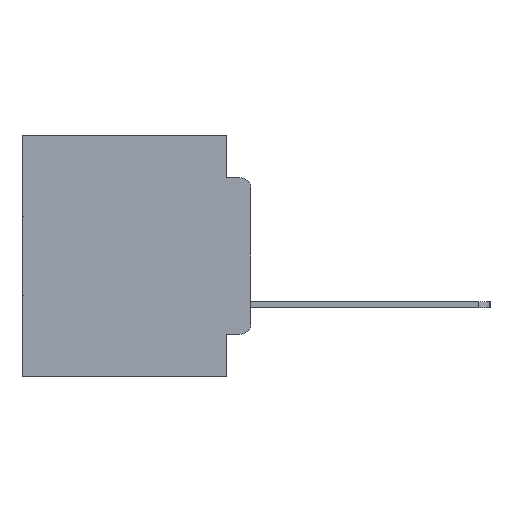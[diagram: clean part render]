
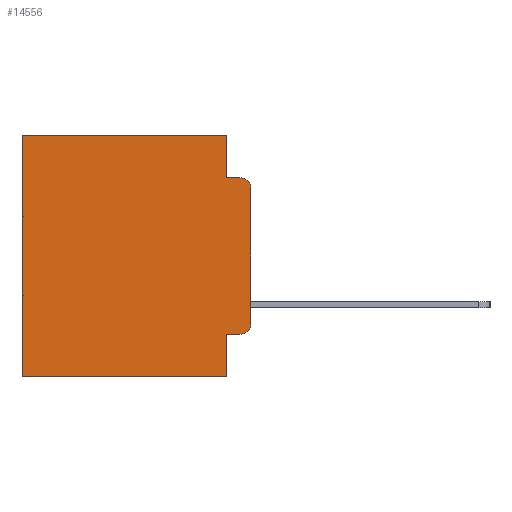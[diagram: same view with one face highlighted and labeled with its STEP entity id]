
A CAD part, left-side view. The second image highlights one B-rep face of the part: STEP entity #14556.
In plain terms, the highlighted planar face has unit normal (-1, 0, 0).
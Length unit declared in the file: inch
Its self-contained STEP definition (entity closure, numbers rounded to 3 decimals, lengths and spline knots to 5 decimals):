
#582 = DIRECTION ( 'NONE',  ( 0., 1., 0. ) ) ;
#583 = EDGE_CURVE ( 'NONE', #15715, #18864, #4426, .T. ) ;
#731 = DIRECTION ( 'NONE',  ( 0., 1., 0. ) ) ;
#733 = CARTESIAN_POINT ( 'NONE',  ( 0.298, 0.051, 0. ) ) ;
#895 = CARTESIAN_POINT ( 'NONE',  ( 0.298, 0., -0.1085 ) ) ;
#943 = VERTEX_POINT ( 'NONE', #2730 ) ;
#1079 = EDGE_CURVE ( 'NONE', #31131, #10600, #2336, .T. ) ;
#2021 = CIRCLE ( 'NONE', #30266, 0.02 ) ;
#2336 = LINE ( 'NONE', #27805, #15197 ) ;
#2464 = VECTOR ( 'NONE', #27382, 39.37008 ) ;
#2730 = CARTESIAN_POINT ( 'NONE',  ( 0.298, 0.051, -0.4115 ) ) ;
#2847 = CARTESIAN_POINT ( 'NONE',  ( 0.298, 0., 0. ) ) ;
#3162 = CARTESIAN_POINT ( 'NONE',  ( 0.298, 0.051, -0.0885 ) ) ;
#3260 = EDGE_CURVE ( 'NONE', #7310, #29753, #29062, .T. ) ;
#3595 = LINE ( 'NONE', #3162, #22775 ) ;
#3669 = CARTESIAN_POINT ( 'NONE',  ( 0.298, 0.02, -0.3915 ) ) ;
#4253 = LINE ( 'NONE', #20819, #9520 ) ;
#4426 = CIRCLE ( 'NONE', #10584, 0.02 ) ;
#4541 = VERTEX_POINT ( 'NONE', #14952 ) ;
#5326 = CARTESIAN_POINT ( 'NONE',  ( 0.298, 0.473, 0. ) ) ;
#6144 = ORIENTED_EDGE ( 'NONE', *, *, #11059, .F. ) ;
#6248 = DIRECTION ( 'NONE',  ( 0., 0., -1. ) ) ;
#7310 = VERTEX_POINT ( 'NONE', #733 ) ;
#7801 = ORIENTED_EDGE ( 'NONE', *, *, #29323, .F. ) ;
#7967 = DIRECTION ( 'NONE',  ( 0., 0., -1. ) ) ;
#8221 = ORIENTED_EDGE ( 'NONE', *, *, #8280, .T. ) ;
#8280 = EDGE_CURVE ( 'NONE', #4541, #8493, #2021, .T. ) ;
#8493 = VERTEX_POINT ( 'NONE', #19785 ) ;
#9520 = VECTOR ( 'NONE', #27814, 39.37008 ) ;
#10584 = AXIS2_PLACEMENT_3D ( 'NONE', #11131, #27946, #13663 ) ;
#10600 = VERTEX_POINT ( 'NONE', #13316 ) ;
#10605 = CARTESIAN_POINT ( 'NONE',  ( 0.298, 0.051, 0. ) ) ;
#10938 = DIRECTION ( 'NONE',  ( 0., -1., 0. ) ) ;
#11059 = EDGE_CURVE ( 'NONE', #15715, #8493, #15126, .T. ) ;
#11131 = CARTESIAN_POINT ( 'NONE',  ( 0.298, 0.02, -0.1085 ) ) ;
#11351 = CARTESIAN_POINT ( 'NONE',  ( 0.298, 0., 0. ) ) ;
#11785 = VECTOR ( 'NONE', #7967, 39.37008 ) ;
#13316 = CARTESIAN_POINT ( 'NONE',  ( 0.298, 0.473, -0.5 ) ) ;
#13372 = ORIENTED_EDGE ( 'NONE', *, *, #16721, .F. ) ;
#13663 = DIRECTION ( 'NONE',  ( 0., 0., -1. ) ) ;
#14172 = FACE_OUTER_BOUND ( 'NONE', #15162, .T. ) ;
#14556 = ADVANCED_FACE ( 'NONE', ( #14172 ), #25851, .F. ) ;
#14952 = CARTESIAN_POINT ( 'NONE',  ( 0.298, 0.02, -0.4115 ) ) ;
#15094 = EDGE_CURVE ( 'NONE', #943, #4541, #28623, .T. ) ;
#15126 = LINE ( 'NONE', #2847, #27010 ) ;
#15162 = EDGE_LOOP ( 'NONE', ( #6144, #26514, #7801, #28649, #23995, #19202, #31545, #13372, #26885, #8221 ) ) ;
#15197 = VECTOR ( 'NONE', #731, 39.37008 ) ;
#15596 = DIRECTION ( 'NONE',  ( 0., 0., -1. ) ) ;
#15715 = VERTEX_POINT ( 'NONE', #895 ) ;
#16399 = DIRECTION ( 'NONE',  ( 0., 0., -1. ) ) ;
#16721 = EDGE_CURVE ( 'NONE', #943, #31131, #4253, .T. ) ;
#17311 = VERTEX_POINT ( 'NONE', #24981 ) ;
#17677 = LINE ( 'NONE', #5326, #11785 ) ;
#18404 = EDGE_CURVE ( 'NONE', #29753, #10600, #17677, .T. ) ;
#18864 = VERTEX_POINT ( 'NONE', #26640 ) ;
#19202 = ORIENTED_EDGE ( 'NONE', *, *, #18404, .T. ) ;
#19785 = CARTESIAN_POINT ( 'NONE',  ( 0.298, 0., -0.3915 ) ) ;
#19989 = AXIS2_PLACEMENT_3D ( 'NONE', #11351, #30465, #16399 ) ;
#20384 = CARTESIAN_POINT ( 'NONE',  ( 0.298, 0.051, -0.4115 ) ) ;
#20819 = CARTESIAN_POINT ( 'NONE',  ( 0.298, 0.051, 0. ) ) ;
#21248 = DIRECTION ( 'NONE',  ( -1., 0., 0. ) ) ;
#21695 = VECTOR ( 'NONE', #29697, 39.37008 ) ;
#22775 = VECTOR ( 'NONE', #10938, 39.37008 ) ;
#22968 = VECTOR ( 'NONE', #582, 39.37008 ) ;
#23179 = CARTESIAN_POINT ( 'NONE',  ( 0.298, 0., 0. ) ) ;
#23995 = ORIENTED_EDGE ( 'NONE', *, *, #3260, .T. ) ;
#24604 = CARTESIAN_POINT ( 'NONE',  ( 0.298, 0.051, -0.5 ) ) ;
#24981 = CARTESIAN_POINT ( 'NONE',  ( 0.298, 0.051, -0.0885 ) ) ;
#25851 = PLANE ( 'NONE',  #19989 ) ;
#26514 = ORIENTED_EDGE ( 'NONE', *, *, #583, .T. ) ;
#26640 = CARTESIAN_POINT ( 'NONE',  ( 0.298, 0.02, -0.0885 ) ) ;
#26681 = CARTESIAN_POINT ( 'NONE',  ( 0.298, 0.473, 0. ) ) ;
#26885 = ORIENTED_EDGE ( 'NONE', *, *, #15094, .T. ) ;
#27010 = VECTOR ( 'NONE', #15596, 39.37008 ) ;
#27382 = DIRECTION ( 'NONE',  ( 0., -1., 0. ) ) ;
#27784 = EDGE_CURVE ( 'NONE', #7310, #17311, #27836, .T. ) ;
#27805 = CARTESIAN_POINT ( 'NONE',  ( 0.298, 0., -0.5 ) ) ;
#27814 = DIRECTION ( 'NONE',  ( 0., 0., -1. ) ) ;
#27836 = LINE ( 'NONE', #10605, #21695 ) ;
#27946 = DIRECTION ( 'NONE',  ( -1., 0., 0. ) ) ;
#28623 = LINE ( 'NONE', #20384, #2464 ) ;
#28649 = ORIENTED_EDGE ( 'NONE', *, *, #27784, .F. ) ;
#29062 = LINE ( 'NONE', #23179, #22968 ) ;
#29323 = EDGE_CURVE ( 'NONE', #17311, #18864, #3595, .T. ) ;
#29697 = DIRECTION ( 'NONE',  ( 0., 0., -1. ) ) ;
#29753 = VERTEX_POINT ( 'NONE', #26681 ) ;
#30266 = AXIS2_PLACEMENT_3D ( 'NONE', #3669, #21248, #6248 ) ;
#30465 = DIRECTION ( 'NONE',  ( 1., 0., 0. ) ) ;
#31131 = VERTEX_POINT ( 'NONE', #24604 ) ;
#31545 = ORIENTED_EDGE ( 'NONE', *, *, #1079, .F. ) ;
